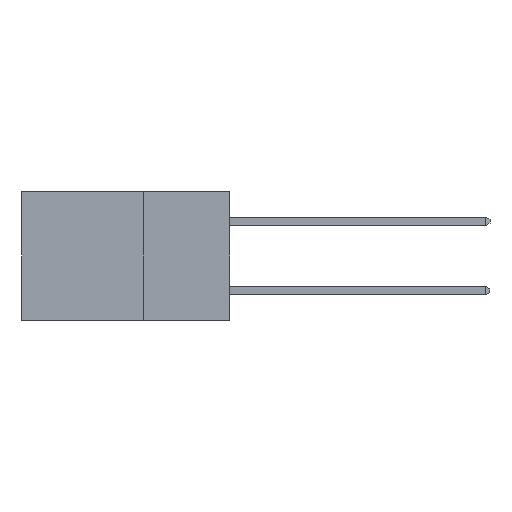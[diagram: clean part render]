
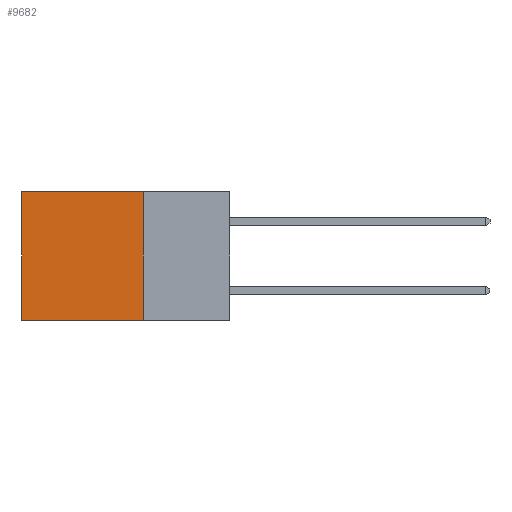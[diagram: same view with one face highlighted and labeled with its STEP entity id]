
A CAD part, left-side view. The second image highlights one B-rep face of the part: STEP entity #9682.
In plain terms, the highlighted planar face has unit normal (-1, 0, 0).
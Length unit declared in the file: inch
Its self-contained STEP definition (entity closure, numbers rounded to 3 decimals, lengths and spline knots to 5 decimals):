
#608 = PLANE ( 'NONE',  #9868 ) ;
#1102 = VERTEX_POINT ( 'NONE', #3471 ) ;
#1107 = ORIENTED_EDGE ( 'NONE', *, *, #5473, .F. ) ;
#1755 = VERTEX_POINT ( 'NONE', #4113 ) ;
#1820 = DIRECTION ( 'NONE',  ( 1., 0., 0. ) ) ;
#2158 = VECTOR ( 'NONE', #12852, 39.37008 ) ;
#2594 = VECTOR ( 'NONE', #9461, 39.37008 ) ;
#3165 = CARTESIAN_POINT ( 'NONE',  ( 0.298, 0.25, 0. ) ) ;
#3263 = DIRECTION ( 'NONE',  ( 0., 1., 0. ) ) ;
#3471 = CARTESIAN_POINT ( 'NONE',  ( 0.298, 0.25, 0. ) ) ;
#4113 = CARTESIAN_POINT ( 'NONE',  ( 0.298, 0.6, -0.37 ) ) ;
#4990 = LINE ( 'NONE', #10294, #8163 ) ;
#5251 = LINE ( 'NONE', #12010, #2158 ) ;
#5473 = EDGE_CURVE ( 'NONE', #1102, #12843, #11889, .T. ) ;
#5513 = EDGE_CURVE ( 'NONE', #8834, #1755, #5251, .T. ) ;
#5517 = DIRECTION ( 'NONE',  ( 0., 0., -1. ) ) ;
#5892 = CARTESIAN_POINT ( 'NONE',  ( 0.298, 0.25, -0.37 ) ) ;
#6237 = ORIENTED_EDGE ( 'NONE', *, *, #5513, .T. ) ;
#8163 = VECTOR ( 'NONE', #3263, 39.37008 ) ;
#8834 = VERTEX_POINT ( 'NONE', #12925 ) ;
#8860 = CARTESIAN_POINT ( 'NONE',  ( 0.298, 0.25, 0. ) ) ;
#9133 = VECTOR ( 'NONE', #5517, 39.37008 ) ;
#9461 = DIRECTION ( 'NONE',  ( 0., 1., 0. ) ) ;
#9682 = ADVANCED_FACE ( 'NONE', ( #10162 ), #608, .F. ) ;
#9834 = EDGE_CURVE ( 'NONE', #1102, #8834, #4990, .T. ) ;
#9868 = AXIS2_PLACEMENT_3D ( 'NONE', #8860, #1820, #10044 ) ;
#10044 = DIRECTION ( 'NONE',  ( 0., 0., -1. ) ) ;
#10162 = FACE_OUTER_BOUND ( 'NONE', #14284, .T. ) ;
#10294 = CARTESIAN_POINT ( 'NONE',  ( 0.298, 0.25, 0. ) ) ;
#10884 = ORIENTED_EDGE ( 'NONE', *, *, #9834, .T. ) ;
#11493 = EDGE_CURVE ( 'NONE', #12843, #1755, #14992, .T. ) ;
#11783 = CARTESIAN_POINT ( 'NONE',  ( 0.298, 0.25, -0.37 ) ) ;
#11889 = LINE ( 'NONE', #3165, #9133 ) ;
#12010 = CARTESIAN_POINT ( 'NONE',  ( 0.298, 0.6, 0. ) ) ;
#12843 = VERTEX_POINT ( 'NONE', #11783 ) ;
#12852 = DIRECTION ( 'NONE',  ( 0., 0., -1. ) ) ;
#12878 = ORIENTED_EDGE ( 'NONE', *, *, #11493, .F. ) ;
#12925 = CARTESIAN_POINT ( 'NONE',  ( 0.298, 0.6, 0. ) ) ;
#14284 = EDGE_LOOP ( 'NONE', ( #6237, #12878, #1107, #10884 ) ) ;
#14992 = LINE ( 'NONE', #5892, #2594 ) ;
